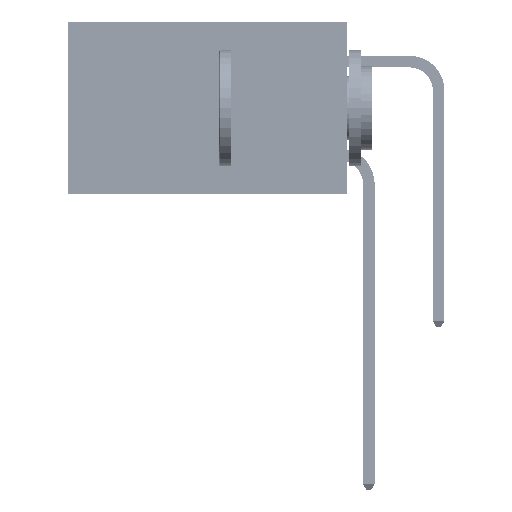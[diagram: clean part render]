
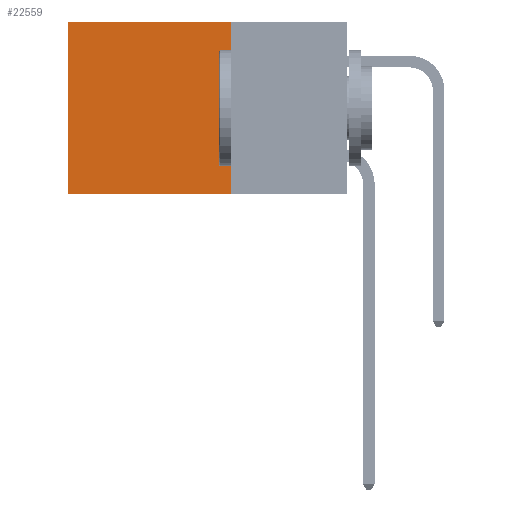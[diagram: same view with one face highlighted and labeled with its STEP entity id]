
A CAD part, left-side view. The second image highlights one B-rep face of the part: STEP entity #22559.
In plain terms, the highlighted planar face has unit normal (-1, 0, 0).
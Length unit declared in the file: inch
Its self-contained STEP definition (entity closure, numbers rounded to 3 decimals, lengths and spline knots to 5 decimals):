
#635 = CARTESIAN_POINT ( 'NONE',  ( 0.2875, 0.25, -0.37 ) ) ;
#1189 = DIRECTION ( 'NONE',  ( 0., 1., 0. ) ) ;
#3469 = EDGE_LOOP ( 'NONE', ( #14506, #46548, #41284, #26830 ) ) ;
#4168 = FACE_OUTER_BOUND ( 'NONE', #3469, .T. ) ;
#5178 = DIRECTION ( 'NONE',  ( 0., 1., 0. ) ) ;
#6778 = CARTESIAN_POINT ( 'NONE',  ( 0.2875, 0.6, 0. ) ) ;
#7776 = CARTESIAN_POINT ( 'NONE',  ( 0.2875, 0.6, -0.37 ) ) ;
#10231 = DIRECTION ( 'NONE',  ( 0., 0., -1. ) ) ;
#14506 = ORIENTED_EDGE ( 'NONE', *, *, #51634, .T. ) ;
#14556 = CARTESIAN_POINT ( 'NONE',  ( 0.2875, 0.25, 0. ) ) ;
#15191 = DIRECTION ( 'NONE',  ( 0., 0., -1. ) ) ;
#16415 = LINE ( 'NONE', #17623, #41959 ) ;
#17623 = CARTESIAN_POINT ( 'NONE',  ( 0.2875, 0.25, 0. ) ) ;
#19177 = CARTESIAN_POINT ( 'NONE',  ( 0.2875, 0.6, 0. ) ) ;
#22063 = VERTEX_POINT ( 'NONE', #38603 ) ;
#22559 = ADVANCED_FACE ( 'NONE', ( #4168 ), #27277, .F. ) ;
#26830 = ORIENTED_EDGE ( 'NONE', *, *, #31021, .T. ) ;
#27117 = VERTEX_POINT ( 'NONE', #19177 ) ;
#27277 = PLANE ( 'NONE',  #33138 ) ;
#30645 = VERTEX_POINT ( 'NONE', #7776 ) ;
#31021 = EDGE_CURVE ( 'NONE', #44662, #27117, #16415, .T. ) ;
#31404 = DIRECTION ( 'NONE',  ( 0., 0., -1. ) ) ;
#32677 = VECTOR ( 'NONE', #5178, 39.37008 ) ;
#33138 = AXIS2_PLACEMENT_3D ( 'NONE', #52078, #43538, #10231 ) ;
#33925 = VECTOR ( 'NONE', #15191, 39.37008 ) ;
#38603 = CARTESIAN_POINT ( 'NONE',  ( 0.2875, 0.25, -0.37 ) ) ;
#39657 = CARTESIAN_POINT ( 'NONE',  ( 0.2875, 0.25, 0. ) ) ;
#41284 = ORIENTED_EDGE ( 'NONE', *, *, #45816, .F. ) ;
#41743 = EDGE_CURVE ( 'NONE', #22063, #30645, #42517, .T. ) ;
#41959 = VECTOR ( 'NONE', #1189, 39.37008 ) ;
#42517 = LINE ( 'NONE', #635, #32677 ) ;
#43538 = DIRECTION ( 'NONE',  ( 1., 0., 0. ) ) ;
#44662 = VERTEX_POINT ( 'NONE', #39657 ) ;
#45816 = EDGE_CURVE ( 'NONE', #44662, #22063, #46531, .T. ) ;
#46531 = LINE ( 'NONE', #14556, #49749 ) ;
#46548 = ORIENTED_EDGE ( 'NONE', *, *, #41743, .F. ) ;
#48956 = LINE ( 'NONE', #6778, #33925 ) ;
#49749 = VECTOR ( 'NONE', #31404, 39.37008 ) ;
#51634 = EDGE_CURVE ( 'NONE', #27117, #30645, #48956, .T. ) ;
#52078 = CARTESIAN_POINT ( 'NONE',  ( 0.2875, 0.25, 0. ) ) ;
